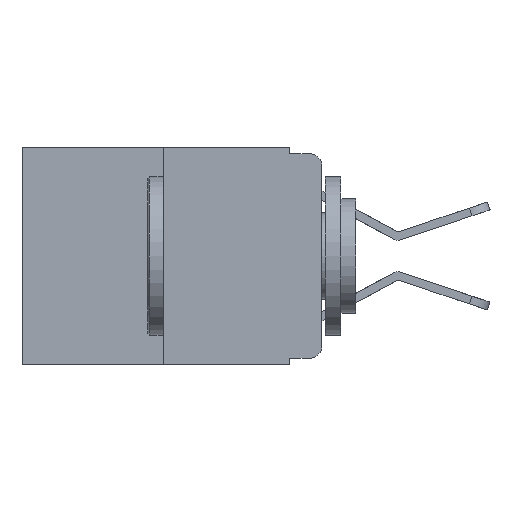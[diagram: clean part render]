
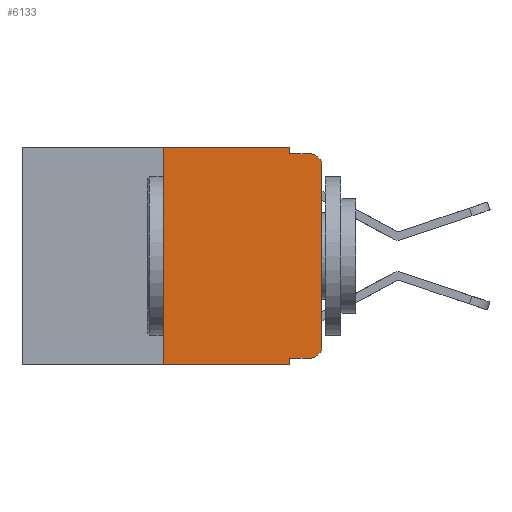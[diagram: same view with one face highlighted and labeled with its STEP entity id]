
A CAD part, left-side view. The second image highlights one B-rep face of the part: STEP entity #6133.
In plain terms, the highlighted planar face has unit normal (-1, 0, 0).
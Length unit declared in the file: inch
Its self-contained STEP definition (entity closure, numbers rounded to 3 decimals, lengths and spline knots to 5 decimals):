
#69 = ORIENTED_EDGE ( 'NONE', *, *, #12157, .F. ) ;
#76 = DIRECTION ( 'NONE',  ( 0., -1., 0. ) ) ;
#99 = CARTESIAN_POINT ( 'NONE',  ( 0., 0.051, -0.333 ) ) ;
#258 = EDGE_CURVE ( 'NONE', #10159, #9990, #5985, .T. ) ;
#316 = FACE_OUTER_BOUND ( 'NONE', #5762, .T. ) ;
#828 = VECTOR ( 'NONE', #3630, 39.37008 ) ;
#985 = VECTOR ( 'NONE', #4247, 39.37008 ) ;
#1087 = VERTEX_POINT ( 'NONE', #8352 ) ;
#1209 = VECTOR ( 'NONE', #10086, 39.37008 ) ;
#1399 = DIRECTION ( 'NONE',  ( -1., 0., 0. ) ) ;
#1523 = LINE ( 'NONE', #12022, #1209 ) ;
#1619 = EDGE_CURVE ( 'NONE', #12065, #8748, #11643, .T. ) ;
#1620 = LINE ( 'NONE', #9076, #985 ) ;
#1694 = EDGE_CURVE ( 'NONE', #1087, #4744, #11337, .T. ) ;
#1870 = VERTEX_POINT ( 'NONE', #7282 ) ;
#1880 = AXIS2_PLACEMENT_3D ( 'NONE', #12685, #1984, #8897 ) ;
#1984 = DIRECTION ( 'NONE',  ( 1., 0., 0. ) ) ;
#2021 = VERTEX_POINT ( 'NONE', #9028 ) ;
#2086 = AXIS2_PLACEMENT_3D ( 'NONE', #7367, #1399, #8339 ) ;
#2105 = ORIENTED_EDGE ( 'NONE', *, *, #9288, .F. ) ;
#2254 = ORIENTED_EDGE ( 'NONE', *, *, #258, .T. ) ;
#2792 = ORIENTED_EDGE ( 'NONE', *, *, #1619, .T. ) ;
#2877 = CARTESIAN_POINT ( 'NONE',  ( 0., 0.051, 0. ) ) ;
#3102 = CIRCLE ( 'NONE', #2086, 0.02 ) ;
#3284 = AXIS2_PLACEMENT_3D ( 'NONE', #11173, #10997, #11159 ) ;
#3630 = DIRECTION ( 'NONE',  ( 0., -1., 0. ) ) ;
#3698 = ORIENTED_EDGE ( 'NONE', *, *, #9594, .F. ) ;
#4001 = CARTESIAN_POINT ( 'NONE',  ( 0., 0.051, -0.333 ) ) ;
#4247 = DIRECTION ( 'NONE',  ( 0., 0., 1. ) ) ;
#4744 = VERTEX_POINT ( 'NONE', #5377 ) ;
#4992 = VERTEX_POINT ( 'NONE', #7708 ) ;
#5012 = LINE ( 'NONE', #2877, #9543 ) ;
#5162 = EDGE_CURVE ( 'NONE', #1087, #1870, #1620, .T. ) ;
#5283 = DIRECTION ( 'NONE',  ( 0., 0., 1. ) ) ;
#5377 = CARTESIAN_POINT ( 'NONE',  ( 0., 0.051, -0.343 ) ) ;
#5585 = ORIENTED_EDGE ( 'NONE', *, *, #12473, .F. ) ;
#5762 = EDGE_LOOP ( 'NONE', ( #11632, #2254, #5585, #3698, #69, #9056, #11595, #2105, #2792, #11943 ) ) ;
#5796 = CARTESIAN_POINT ( 'NONE',  ( 0., 0., -0.03 ) ) ;
#5985 = CIRCLE ( 'NONE', #3284, 0.02 ) ;
#6083 = DIRECTION ( 'NONE',  ( 0., -1., 0. ) ) ;
#6133 = ADVANCED_FACE ( 'NONE', ( #316 ), #11744, .F. ) ;
#6474 = VERTEX_POINT ( 'NONE', #12299 ) ;
#7071 = VECTOR ( 'NONE', #76, 39.37008 ) ;
#7282 = CARTESIAN_POINT ( 'NONE',  ( 0., 0.25, 0. ) ) ;
#7343 = LINE ( 'NONE', #10392, #828 ) ;
#7367 = CARTESIAN_POINT ( 'NONE',  ( 0., 0.02, -0.313 ) ) ;
#7369 = EDGE_CURVE ( 'NONE', #6474, #10159, #11976, .T. ) ;
#7708 = CARTESIAN_POINT ( 'NONE',  ( 0., 0.051, 0. ) ) ;
#7781 = DIRECTION ( 'NONE',  ( 0., 0., -1. ) ) ;
#8160 = CARTESIAN_POINT ( 'NONE',  ( 0., 0., 0. ) ) ;
#8339 = DIRECTION ( 'NONE',  ( 0., 0., -1. ) ) ;
#8352 = CARTESIAN_POINT ( 'NONE',  ( 0., 0.25, -0.343 ) ) ;
#8407 = CARTESIAN_POINT ( 'NONE',  ( 0., 0.02, -0.01 ) ) ;
#8500 = VECTOR ( 'NONE', #6083, 39.37008 ) ;
#8646 = DIRECTION ( 'NONE',  ( 0., -1., 0. ) ) ;
#8748 = VERTEX_POINT ( 'NONE', #8878 ) ;
#8878 = CARTESIAN_POINT ( 'NONE',  ( 0., 0.02, -0.333 ) ) ;
#8897 = DIRECTION ( 'NONE',  ( 0., 0., -1. ) ) ;
#9028 = CARTESIAN_POINT ( 'NONE',  ( 0., 0.051, -0.01 ) ) ;
#9056 = ORIENTED_EDGE ( 'NONE', *, *, #5162, .F. ) ;
#9076 = CARTESIAN_POINT ( 'NONE',  ( 0., 0.25, 0. ) ) ;
#9089 = VECTOR ( 'NONE', #8646, 39.37008 ) ;
#9288 = EDGE_CURVE ( 'NONE', #12065, #4744, #5012, .T. ) ;
#9440 = VECTOR ( 'NONE', #5283, 39.37008 ) ;
#9543 = VECTOR ( 'NONE', #7781, 39.37008 ) ;
#9594 = EDGE_CURVE ( 'NONE', #4992, #2021, #1523, .T. ) ;
#9990 = VERTEX_POINT ( 'NONE', #8407 ) ;
#10086 = DIRECTION ( 'NONE',  ( 0., 0., -1. ) ) ;
#10159 = VERTEX_POINT ( 'NONE', #5796 ) ;
#10392 = CARTESIAN_POINT ( 'NONE',  ( 0., 0.051, -0.01 ) ) ;
#10997 = DIRECTION ( 'NONE',  ( -1., 0., 0. ) ) ;
#11159 = DIRECTION ( 'NONE',  ( 0., 0., -1. ) ) ;
#11173 = CARTESIAN_POINT ( 'NONE',  ( 0., 0.02, -0.03 ) ) ;
#11181 = CARTESIAN_POINT ( 'NONE',  ( 0., 0.473, -0.343 ) ) ;
#11214 = EDGE_CURVE ( 'NONE', #8748, #6474, #3102, .T. ) ;
#11337 = LINE ( 'NONE', #11181, #8500 ) ;
#11595 = ORIENTED_EDGE ( 'NONE', *, *, #1694, .T. ) ;
#11632 = ORIENTED_EDGE ( 'NONE', *, *, #7369, .T. ) ;
#11643 = LINE ( 'NONE', #99, #9089 ) ;
#11744 = PLANE ( 'NONE',  #1880 ) ;
#11830 = CARTESIAN_POINT ( 'NONE',  ( 0., 0.473, 0. ) ) ;
#11943 = ORIENTED_EDGE ( 'NONE', *, *, #11214, .T. ) ;
#11976 = LINE ( 'NONE', #8160, #9440 ) ;
#12022 = CARTESIAN_POINT ( 'NONE',  ( 0., 0.051, 0. ) ) ;
#12065 = VERTEX_POINT ( 'NONE', #4001 ) ;
#12144 = LINE ( 'NONE', #11830, #7071 ) ;
#12157 = EDGE_CURVE ( 'NONE', #1870, #4992, #12144, .T. ) ;
#12299 = CARTESIAN_POINT ( 'NONE',  ( 0., 0., -0.313 ) ) ;
#12473 = EDGE_CURVE ( 'NONE', #2021, #9990, #7343, .T. ) ;
#12685 = CARTESIAN_POINT ( 'NONE',  ( 0., 0.473, 0. ) ) ;
